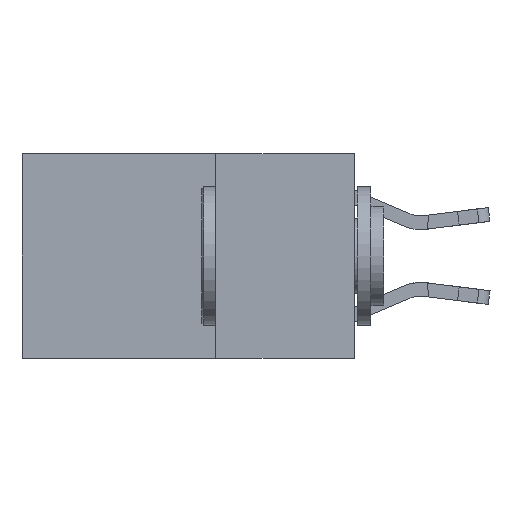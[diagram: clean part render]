
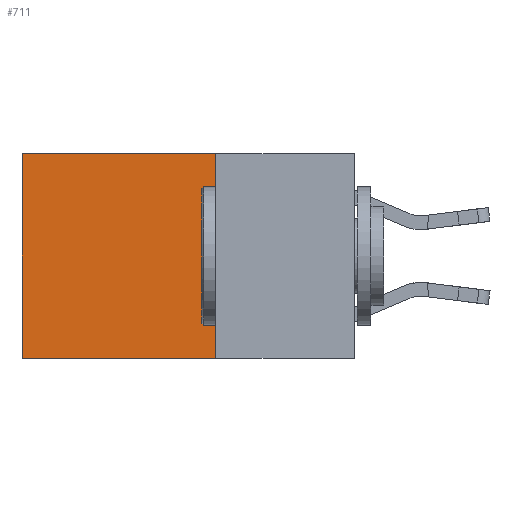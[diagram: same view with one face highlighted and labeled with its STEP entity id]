
A CAD part, left-side view. The second image highlights one B-rep face of the part: STEP entity #711.
In plain terms, the highlighted planar face has unit normal (-1, 0, 0).
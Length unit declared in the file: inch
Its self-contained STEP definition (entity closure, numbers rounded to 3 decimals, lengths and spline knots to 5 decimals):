
#109 = EDGE_CURVE ( 'NONE', #7653, #16690, #12841, .T. ) ;
#711 = ADVANCED_FACE ( 'NONE', ( #15249 ), #5567, .F. ) ;
#1213 = VECTOR ( 'NONE', #22373, 39.37008 ) ;
#1915 = LINE ( 'NONE', #4758, #1213 ) ;
#3819 = ORIENTED_EDGE ( 'NONE', *, *, #10142, .F. ) ;
#4758 = CARTESIAN_POINT ( 'NONE',  ( 0.2625, 0.6, 0. ) ) ;
#5099 = CARTESIAN_POINT ( 'NONE',  ( 0.2625, 0.6, -0.37 ) ) ;
#5567 = PLANE ( 'NONE',  #24283 ) ;
#6927 = VECTOR ( 'NONE', #21476, 39.37008 ) ;
#7653 = VERTEX_POINT ( 'NONE', #11478 ) ;
#8576 = VECTOR ( 'NONE', #13609, 39.37008 ) ;
#10053 = CARTESIAN_POINT ( 'NONE',  ( 0.2625, 0.25, 0. ) ) ;
#10142 = EDGE_CURVE ( 'NONE', #16690, #14516, #14460, .T. ) ;
#11360 = CARTESIAN_POINT ( 'NONE',  ( 0.2625, 0.25, -0.37 ) ) ;
#11478 = CARTESIAN_POINT ( 'NONE',  ( 0.2625, 0.25, 0. ) ) ;
#12268 = DIRECTION ( 'NONE',  ( 1., 0., 0. ) ) ;
#12841 = LINE ( 'NONE', #14924, #6927 ) ;
#13609 = DIRECTION ( 'NONE',  ( 0., 1., 0. ) ) ;
#14460 = LINE ( 'NONE', #11360, #8576 ) ;
#14516 = VERTEX_POINT ( 'NONE', #5099 ) ;
#14924 = CARTESIAN_POINT ( 'NONE',  ( 0.2625, 0.25, 0. ) ) ;
#15249 = FACE_OUTER_BOUND ( 'NONE', #22027, .T. ) ;
#15759 = VERTEX_POINT ( 'NONE', #24547 ) ;
#16369 = CARTESIAN_POINT ( 'NONE',  ( 0.2625, 0.25, 0. ) ) ;
#16485 = EDGE_CURVE ( 'NONE', #7653, #15759, #21378, .T. ) ;
#16690 = VERTEX_POINT ( 'NONE', #19164 ) ;
#18529 = DIRECTION ( 'NONE',  ( 0., 1., 0. ) ) ;
#19164 = CARTESIAN_POINT ( 'NONE',  ( 0.2625, 0.25, -0.37 ) ) ;
#19881 = ORIENTED_EDGE ( 'NONE', *, *, #109, .F. ) ;
#20696 = VECTOR ( 'NONE', #18529, 39.37008 ) ;
#21378 = LINE ( 'NONE', #16369, #20696 ) ;
#21476 = DIRECTION ( 'NONE',  ( 0., 0., -1. ) ) ;
#22027 = EDGE_LOOP ( 'NONE', ( #26291, #3819, #19881, #22701 ) ) ;
#22373 = DIRECTION ( 'NONE',  ( 0., 0., -1. ) ) ;
#22701 = ORIENTED_EDGE ( 'NONE', *, *, #16485, .T. ) ;
#24283 = AXIS2_PLACEMENT_3D ( 'NONE', #10053, #12268, #27541 ) ;
#24547 = CARTESIAN_POINT ( 'NONE',  ( 0.2625, 0.6, 0. ) ) ;
#26291 = ORIENTED_EDGE ( 'NONE', *, *, #27339, .T. ) ;
#27339 = EDGE_CURVE ( 'NONE', #15759, #14516, #1915, .T. ) ;
#27541 = DIRECTION ( 'NONE',  ( 0., 0., -1. ) ) ;
